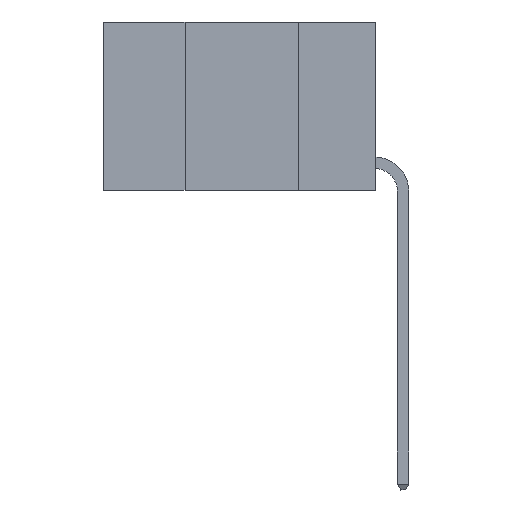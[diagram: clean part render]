
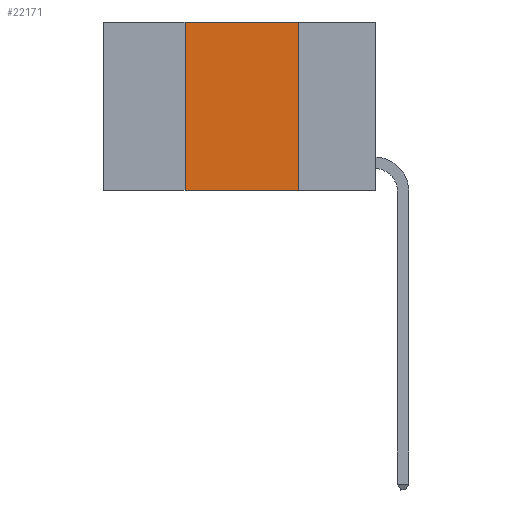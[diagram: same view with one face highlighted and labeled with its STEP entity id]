
A CAD part, left-side view. The second image highlights one B-rep face of the part: STEP entity #22171.
In plain terms, the highlighted planar face has unit normal (-1, 0, 0).
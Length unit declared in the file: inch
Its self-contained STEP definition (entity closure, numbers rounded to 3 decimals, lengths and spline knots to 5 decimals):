
#98 = DIRECTION ( 'NONE',  ( 0., 0., -1. ) ) ;
#1223 = DIRECTION ( 'NONE',  ( 1., 0., 0. ) ) ;
#1359 = CARTESIAN_POINT ( 'NONE',  ( 0., 0.6, -0.37 ) ) ;
#3629 = EDGE_LOOP ( 'NONE', ( #26713, #8833, #5550, #18753 ) ) ;
#5550 = ORIENTED_EDGE ( 'NONE', *, *, #23039, .F. ) ;
#5814 = PLANE ( 'NONE',  #25554 ) ;
#6038 = DIRECTION ( 'NONE',  ( 0., -1., 0. ) ) ;
#6626 = LINE ( 'NONE', #7489, #12830 ) ;
#7489 = CARTESIAN_POINT ( 'NONE',  ( 0., 0.42, 0. ) ) ;
#7814 = VECTOR ( 'NONE', #10482, 39.37008 ) ;
#8537 = LINE ( 'NONE', #15115, #7814 ) ;
#8833 = ORIENTED_EDGE ( 'NONE', *, *, #20855, .F. ) ;
#8920 = VERTEX_POINT ( 'NONE', #22113 ) ;
#9207 = VERTEX_POINT ( 'NONE', #16242 ) ;
#9474 = VECTOR ( 'NONE', #6038, 39.37008 ) ;
#10482 = DIRECTION ( 'NONE',  ( 0., -1., 0. ) ) ;
#10660 = LINE ( 'NONE', #21133, #22344 ) ;
#11052 = CARTESIAN_POINT ( 'NONE',  ( 0., 0.42, -0.37 ) ) ;
#12567 = EDGE_CURVE ( 'NONE', #9207, #8920, #10660, .T. ) ;
#12830 = VECTOR ( 'NONE', #21474, 39.37008 ) ;
#12892 = FACE_OUTER_BOUND ( 'NONE', #3629, .T. ) ;
#15115 = CARTESIAN_POINT ( 'NONE',  ( 0., 0.6, 0. ) ) ;
#16242 = CARTESIAN_POINT ( 'NONE',  ( 0., 0.17, 0. ) ) ;
#17579 = DIRECTION ( 'NONE',  ( 0., 0., -1. ) ) ;
#17813 = EDGE_CURVE ( 'NONE', #21663, #8920, #28078, .T. ) ;
#18753 = ORIENTED_EDGE ( 'NONE', *, *, #17813, .T. ) ;
#18956 = VERTEX_POINT ( 'NONE', #26482 ) ;
#20855 = EDGE_CURVE ( 'NONE', #18956, #9207, #8537, .T. ) ;
#21133 = CARTESIAN_POINT ( 'NONE',  ( 0., 0.17, 0. ) ) ;
#21474 = DIRECTION ( 'NONE',  ( 0., 0., 1. ) ) ;
#21663 = VERTEX_POINT ( 'NONE', #11052 ) ;
#22113 = CARTESIAN_POINT ( 'NONE',  ( 0., 0.17, -0.37 ) ) ;
#22171 = ADVANCED_FACE ( 'NONE', ( #12892 ), #5814, .F. ) ;
#22344 = VECTOR ( 'NONE', #98, 39.37008 ) ;
#23039 = EDGE_CURVE ( 'NONE', #21663, #18956, #6626, .T. ) ;
#25554 = AXIS2_PLACEMENT_3D ( 'NONE', #26823, #1223, #17579 ) ;
#26482 = CARTESIAN_POINT ( 'NONE',  ( 0., 0.42, 0. ) ) ;
#26713 = ORIENTED_EDGE ( 'NONE', *, *, #12567, .F. ) ;
#26823 = CARTESIAN_POINT ( 'NONE',  ( 0., 0.6, 0. ) ) ;
#28078 = LINE ( 'NONE', #1359, #9474 ) ;
